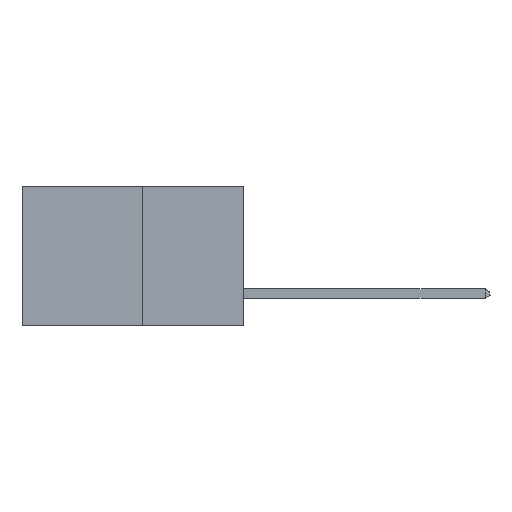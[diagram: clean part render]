
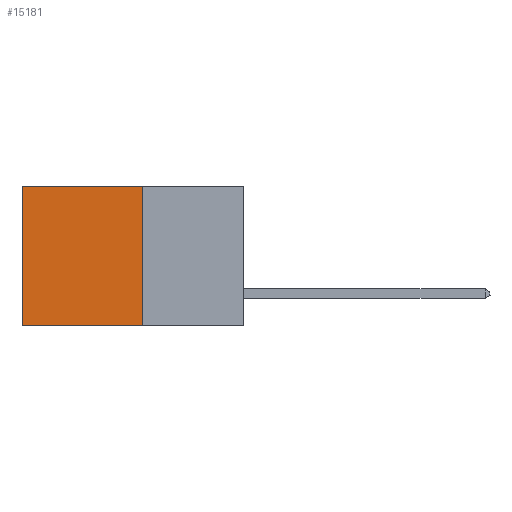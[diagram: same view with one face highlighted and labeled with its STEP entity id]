
A CAD part, left-side view. The second image highlights one B-rep face of the part: STEP entity #15181.
In plain terms, the highlighted planar face has unit normal (-1, 0, 0).
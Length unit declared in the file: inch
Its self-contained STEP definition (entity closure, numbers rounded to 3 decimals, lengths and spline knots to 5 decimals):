
#719 = CARTESIAN_POINT ( 'NONE',  ( 0.277, 0.59, 0. ) ) ;
#1460 = CARTESIAN_POINT ( 'NONE',  ( 0.277, 0.27, 0. ) ) ;
#1523 = EDGE_CURVE ( 'NONE', #1880, #9669, #16816, .T. ) ;
#1548 = DIRECTION ( 'NONE',  ( 0., 0., -1. ) ) ;
#1880 = VERTEX_POINT ( 'NONE', #1460 ) ;
#3133 = EDGE_LOOP ( 'NONE', ( #12480, #8039, #12369, #12125 ) ) ;
#4158 = CARTESIAN_POINT ( 'NONE',  ( 0.277, 0.59, -0.37 ) ) ;
#4179 = CARTESIAN_POINT ( 'NONE',  ( 0.277, 0.27, -0.37 ) ) ;
#4640 = CARTESIAN_POINT ( 'NONE',  ( 0.277, 0.27, -0.37 ) ) ;
#4785 = CARTESIAN_POINT ( 'NONE',  ( 0.277, 0.27, -0.37 ) ) ;
#4847 = DIRECTION ( 'NONE',  ( 0., 0., -1. ) ) ;
#6103 = DIRECTION ( 'NONE',  ( 0., 0., -1. ) ) ;
#6344 = VECTOR ( 'NONE', #4847, 39.37008 ) ;
#6420 = VERTEX_POINT ( 'NONE', #719 ) ;
#7388 = PLANE ( 'NONE',  #10169 ) ;
#8039 = ORIENTED_EDGE ( 'NONE', *, *, #11334, .F. ) ;
#8939 = EDGE_CURVE ( 'NONE', #1880, #6420, #10704, .T. ) ;
#9237 = DIRECTION ( 'NONE',  ( 0., 1., 0. ) ) ;
#9414 = VECTOR ( 'NONE', #16146, 39.37008 ) ;
#9669 = VERTEX_POINT ( 'NONE', #4640 ) ;
#10169 = AXIS2_PLACEMENT_3D ( 'NONE', #4785, #13930, #6103 ) ;
#10292 = VECTOR ( 'NONE', #9237, 39.37008 ) ;
#10543 = CARTESIAN_POINT ( 'NONE',  ( 0.277, 0.27, 0. ) ) ;
#10704 = LINE ( 'NONE', #10543, #10292 ) ;
#11334 = EDGE_CURVE ( 'NONE', #9669, #11708, #16467, .T. ) ;
#11708 = VERTEX_POINT ( 'NONE', #16920 ) ;
#11943 = EDGE_CURVE ( 'NONE', #6420, #11708, #16651, .T. ) ;
#12089 = CARTESIAN_POINT ( 'NONE',  ( 0.277, 0.27, -0.37 ) ) ;
#12125 = ORIENTED_EDGE ( 'NONE', *, *, #8939, .T. ) ;
#12369 = ORIENTED_EDGE ( 'NONE', *, *, #1523, .F. ) ;
#12480 = ORIENTED_EDGE ( 'NONE', *, *, #11943, .T. ) ;
#13123 = VECTOR ( 'NONE', #1548, 39.37008 ) ;
#13765 = FACE_OUTER_BOUND ( 'NONE', #3133, .T. ) ;
#13930 = DIRECTION ( 'NONE',  ( 1., 0., 0. ) ) ;
#15181 = ADVANCED_FACE ( 'NONE', ( #13765 ), #7388, .F. ) ;
#16146 = DIRECTION ( 'NONE',  ( 0., 1., 0. ) ) ;
#16467 = LINE ( 'NONE', #12089, #9414 ) ;
#16651 = LINE ( 'NONE', #4158, #13123 ) ;
#16816 = LINE ( 'NONE', #4179, #6344 ) ;
#16920 = CARTESIAN_POINT ( 'NONE',  ( 0.277, 0.59, -0.37 ) ) ;
